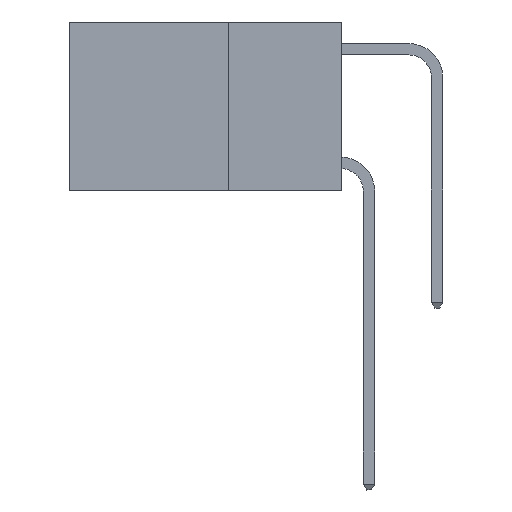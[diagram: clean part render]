
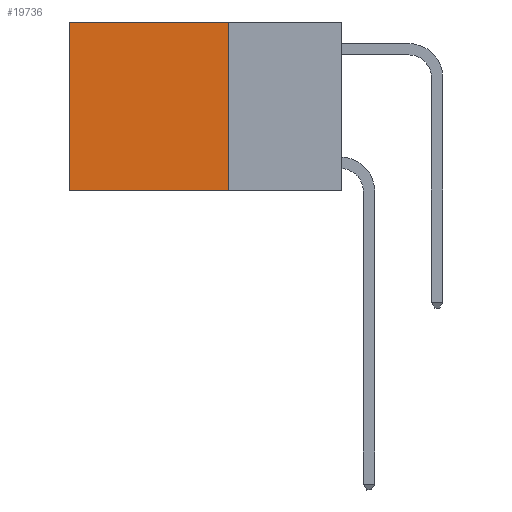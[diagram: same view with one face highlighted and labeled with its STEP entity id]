
A CAD part, left-side view. The second image highlights one B-rep face of the part: STEP entity #19736.
In plain terms, the highlighted planar face has unit normal (-1, 0, 0).
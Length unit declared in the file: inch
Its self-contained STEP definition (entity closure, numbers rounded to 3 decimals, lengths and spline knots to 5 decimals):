
#519 = CARTESIAN_POINT ( 'NONE',  ( 0.2625, 0.6, 0. ) ) ;
#639 = VECTOR ( 'NONE', #22709, 39.37008 ) ;
#2763 = VECTOR ( 'NONE', #11026, 39.37008 ) ;
#3699 = EDGE_CURVE ( 'NONE', #12315, #8859, #13974, .T. ) ;
#3991 = CARTESIAN_POINT ( 'NONE',  ( 0.2625, 0.6, -0.37 ) ) ;
#4797 = ORIENTED_EDGE ( 'NONE', *, *, #3699, .T. ) ;
#5310 = LINE ( 'NONE', #519, #29461 ) ;
#6220 = CARTESIAN_POINT ( 'NONE',  ( 0.2625, 0.25, 0. ) ) ;
#8208 = VERTEX_POINT ( 'NONE', #3991 ) ;
#8756 = VERTEX_POINT ( 'NONE', #19987 ) ;
#8859 = VERTEX_POINT ( 'NONE', #27150 ) ;
#9024 = DIRECTION ( 'NONE',  ( 1., 0., 0. ) ) ;
#10305 = VECTOR ( 'NONE', #14991, 39.37008 ) ;
#11026 = DIRECTION ( 'NONE',  ( 0., 0., -1. ) ) ;
#11118 = ORIENTED_EDGE ( 'NONE', *, *, #13676, .F. ) ;
#11315 = PLANE ( 'NONE',  #20827 ) ;
#12315 = VERTEX_POINT ( 'NONE', #17672 ) ;
#13676 = EDGE_CURVE ( 'NONE', #12315, #8756, #14640, .T. ) ;
#13974 = LINE ( 'NONE', #6220, #639 ) ;
#14157 = EDGE_LOOP ( 'NONE', ( #16127, #15084, #11118, #4797 ) ) ;
#14640 = LINE ( 'NONE', #25030, #2763 ) ;
#14991 = DIRECTION ( 'NONE',  ( 0., 1., 0. ) ) ;
#15084 = ORIENTED_EDGE ( 'NONE', *, *, #17698, .F. ) ;
#16127 = ORIENTED_EDGE ( 'NONE', *, *, #20734, .T. ) ;
#16614 = LINE ( 'NONE', #24276, #10305 ) ;
#17672 = CARTESIAN_POINT ( 'NONE',  ( 0.2625, 0.25, 0. ) ) ;
#17698 = EDGE_CURVE ( 'NONE', #8756, #8208, #16614, .T. ) ;
#19393 = DIRECTION ( 'NONE',  ( 0., 0., -1. ) ) ;
#19736 = ADVANCED_FACE ( 'NONE', ( #25973 ), #11315, .F. ) ;
#19987 = CARTESIAN_POINT ( 'NONE',  ( 0.2625, 0.25, -0.37 ) ) ;
#20734 = EDGE_CURVE ( 'NONE', #8859, #8208, #5310, .T. ) ;
#20827 = AXIS2_PLACEMENT_3D ( 'NONE', #23096, #9024, #25395 ) ;
#22709 = DIRECTION ( 'NONE',  ( 0., 1., 0. ) ) ;
#23096 = CARTESIAN_POINT ( 'NONE',  ( 0.2625, 0.25, 0. ) ) ;
#24276 = CARTESIAN_POINT ( 'NONE',  ( 0.2625, 0.25, -0.37 ) ) ;
#25030 = CARTESIAN_POINT ( 'NONE',  ( 0.2625, 0.25, 0. ) ) ;
#25395 = DIRECTION ( 'NONE',  ( 0., 0., -1. ) ) ;
#25973 = FACE_OUTER_BOUND ( 'NONE', #14157, .T. ) ;
#27150 = CARTESIAN_POINT ( 'NONE',  ( 0.2625, 0.6, 0. ) ) ;
#29461 = VECTOR ( 'NONE', #19393, 39.37008 ) ;
